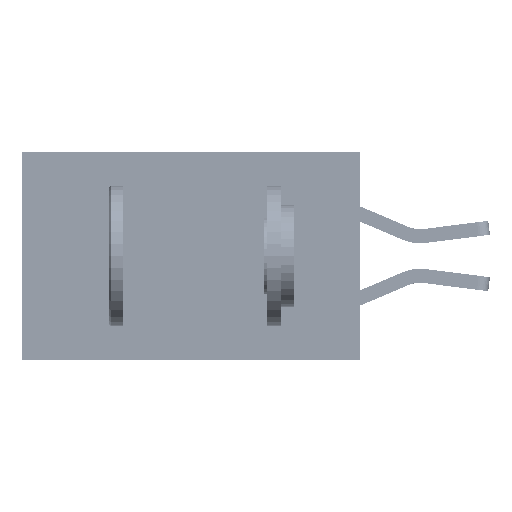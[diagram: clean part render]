
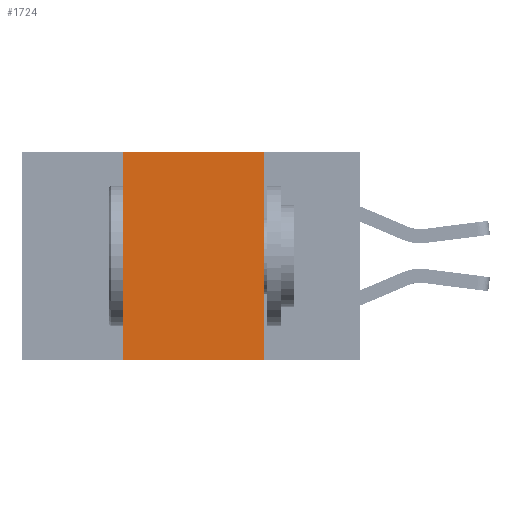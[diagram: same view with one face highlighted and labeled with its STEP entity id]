
A CAD part, left-side view. The second image highlights one B-rep face of the part: STEP entity #1724.
In plain terms, the highlighted planar face has unit normal (-1, 0, 0).
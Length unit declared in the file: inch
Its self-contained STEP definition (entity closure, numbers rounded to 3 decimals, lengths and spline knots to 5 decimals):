
#82 = PLANE ( 'NONE',  #40598 ) ;
#1257 = VERTEX_POINT ( 'NONE', #48941 ) ;
#1724 = ADVANCED_FACE ( 'NONE', ( #43821 ), #82, .F. ) ;
#4530 = LINE ( 'NONE', #17195, #33880 ) ;
#7748 = CARTESIAN_POINT ( 'NONE',  ( 0., 0.6, 0. ) ) ;
#7923 = DIRECTION ( 'NONE',  ( 0., 0., -1. ) ) ;
#8230 = VECTOR ( 'NONE', #8271, 39.37008 ) ;
#8271 = DIRECTION ( 'NONE',  ( 0., 0., -1. ) ) ;
#11412 = DIRECTION ( 'NONE',  ( 1., 0., 0. ) ) ;
#11826 = EDGE_LOOP ( 'NONE', ( #13611, #30962, #42534, #33763 ) ) ;
#13036 = DIRECTION ( 'NONE',  ( 0., -1., 0. ) ) ;
#13611 = ORIENTED_EDGE ( 'NONE', *, *, #42441, .F. ) ;
#14185 = LINE ( 'NONE', #23708, #44710 ) ;
#16031 = CARTESIAN_POINT ( 'NONE',  ( 0., 0.17, 0. ) ) ;
#17195 = CARTESIAN_POINT ( 'NONE',  ( 0., 0.6, -0.37 ) ) ;
#17608 = LINE ( 'NONE', #25245, #43155 ) ;
#19520 = DIRECTION ( 'NONE',  ( 0., 0., 1. ) ) ;
#23708 = CARTESIAN_POINT ( 'NONE',  ( 0., 0.42, 0. ) ) ;
#25245 = CARTESIAN_POINT ( 'NONE',  ( 0., 0.6, 0. ) ) ;
#30962 = ORIENTED_EDGE ( 'NONE', *, *, #34783, .F. ) ;
#31998 = EDGE_CURVE ( 'NONE', #1257, #41885, #4530, .T. ) ;
#33763 = ORIENTED_EDGE ( 'NONE', *, *, #31998, .T. ) ;
#33880 = VECTOR ( 'NONE', #44372, 39.37008 ) ;
#34783 = EDGE_CURVE ( 'NONE', #46459, #36538, #17608, .T. ) ;
#35876 = CARTESIAN_POINT ( 'NONE',  ( 0., 0.17, -0.37 ) ) ;
#36538 = VERTEX_POINT ( 'NONE', #16031 ) ;
#38241 = EDGE_CURVE ( 'NONE', #1257, #46459, #14185, .T. ) ;
#40598 = AXIS2_PLACEMENT_3D ( 'NONE', #7748, #11412, #7923 ) ;
#41296 = LINE ( 'NONE', #48183, #8230 ) ;
#41885 = VERTEX_POINT ( 'NONE', #35876 ) ;
#42441 = EDGE_CURVE ( 'NONE', #36538, #41885, #41296, .T. ) ;
#42534 = ORIENTED_EDGE ( 'NONE', *, *, #38241, .F. ) ;
#43155 = VECTOR ( 'NONE', #13036, 39.37008 ) ;
#43821 = FACE_OUTER_BOUND ( 'NONE', #11826, .T. ) ;
#44372 = DIRECTION ( 'NONE',  ( 0., -1., 0. ) ) ;
#44710 = VECTOR ( 'NONE', #19520, 39.37008 ) ;
#46459 = VERTEX_POINT ( 'NONE', #47279 ) ;
#47279 = CARTESIAN_POINT ( 'NONE',  ( 0., 0.42, 0. ) ) ;
#48183 = CARTESIAN_POINT ( 'NONE',  ( 0., 0.17, 0. ) ) ;
#48941 = CARTESIAN_POINT ( 'NONE',  ( 0., 0.42, -0.37 ) ) ;
